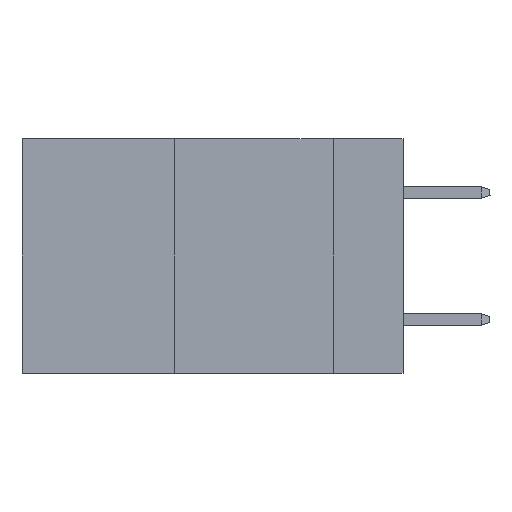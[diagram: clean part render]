
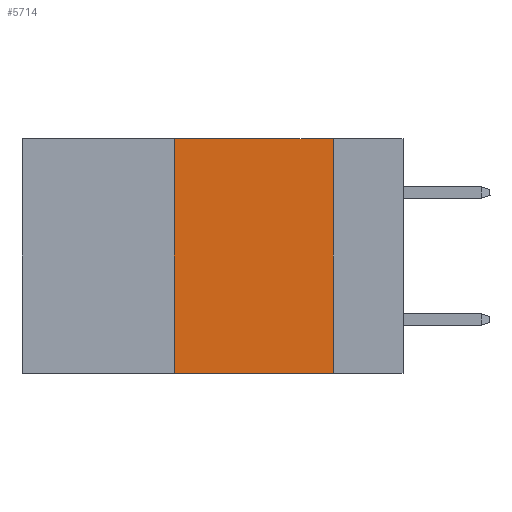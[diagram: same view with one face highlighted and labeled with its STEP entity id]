
A CAD part, left-side view. The second image highlights one B-rep face of the part: STEP entity #5714.
In plain terms, the highlighted planar face has unit normal (-1, 0, 0).
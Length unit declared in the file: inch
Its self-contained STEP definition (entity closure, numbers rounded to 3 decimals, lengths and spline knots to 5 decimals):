
#1015 = DIRECTION ( 'NONE',  ( 0., 0., -1. ) ) ;
#3952 = LINE ( 'NONE', #22237, #19514 ) ;
#5120 = PLANE ( 'NONE',  #14021 ) ;
#5497 = LINE ( 'NONE', #9336, #13157 ) ;
#5714 = ADVANCED_FACE ( 'NONE', ( #26366 ), #5120, .F. ) ;
#7369 = DIRECTION ( 'NONE',  ( 0., -1., 0. ) ) ;
#7984 = EDGE_CURVE ( 'NONE', #23326, #30201, #5497, .T. ) ;
#8507 = DIRECTION ( 'NONE',  ( 0., 0., 1. ) ) ;
#9336 = CARTESIAN_POINT ( 'NONE',  ( 0., 0.6, 0. ) ) ;
#12465 = CARTESIAN_POINT ( 'NONE',  ( 0., 0.6, -0.37 ) ) ;
#13090 = VERTEX_POINT ( 'NONE', #14954 ) ;
#13149 = CARTESIAN_POINT ( 'NONE',  ( 0., 0.36, 0. ) ) ;
#13157 = VECTOR ( 'NONE', #19090, 39.37008 ) ;
#14021 = AXIS2_PLACEMENT_3D ( 'NONE', #17308, #22162, #23877 ) ;
#14624 = EDGE_CURVE ( 'NONE', #30201, #13090, #3952, .T. ) ;
#14954 = CARTESIAN_POINT ( 'NONE',  ( 0., 0.11, -0.37 ) ) ;
#15464 = LINE ( 'NONE', #13149, #17132 ) ;
#16675 = VECTOR ( 'NONE', #7369, 39.37008 ) ;
#16958 = LINE ( 'NONE', #12465, #16675 ) ;
#17043 = EDGE_LOOP ( 'NONE', ( #21751, #27775, #17377, #26650 ) ) ;
#17132 = VECTOR ( 'NONE', #8507, 39.37008 ) ;
#17172 = CARTESIAN_POINT ( 'NONE',  ( 0., 0.36, 0. ) ) ;
#17308 = CARTESIAN_POINT ( 'NONE',  ( 0., 0.6, 0. ) ) ;
#17377 = ORIENTED_EDGE ( 'NONE', *, *, #17394, .F. ) ;
#17394 = EDGE_CURVE ( 'NONE', #22166, #23326, #15464, .T. ) ;
#19090 = DIRECTION ( 'NONE',  ( 0., -1., 0. ) ) ;
#19514 = VECTOR ( 'NONE', #1015, 39.37008 ) ;
#20079 = EDGE_CURVE ( 'NONE', #22166, #13090, #16958, .T. ) ;
#21751 = ORIENTED_EDGE ( 'NONE', *, *, #14624, .F. ) ;
#22162 = DIRECTION ( 'NONE',  ( 1., 0., 0. ) ) ;
#22166 = VERTEX_POINT ( 'NONE', #24620 ) ;
#22237 = CARTESIAN_POINT ( 'NONE',  ( 0., 0.11, 0. ) ) ;
#23326 = VERTEX_POINT ( 'NONE', #17172 ) ;
#23877 = DIRECTION ( 'NONE',  ( 0., 0., -1. ) ) ;
#24620 = CARTESIAN_POINT ( 'NONE',  ( 0., 0.36, -0.37 ) ) ;
#26366 = FACE_OUTER_BOUND ( 'NONE', #17043, .T. ) ;
#26650 = ORIENTED_EDGE ( 'NONE', *, *, #20079, .T. ) ;
#27775 = ORIENTED_EDGE ( 'NONE', *, *, #7984, .F. ) ;
#29956 = CARTESIAN_POINT ( 'NONE',  ( 0., 0.11, 0. ) ) ;
#30201 = VERTEX_POINT ( 'NONE', #29956 ) ;
